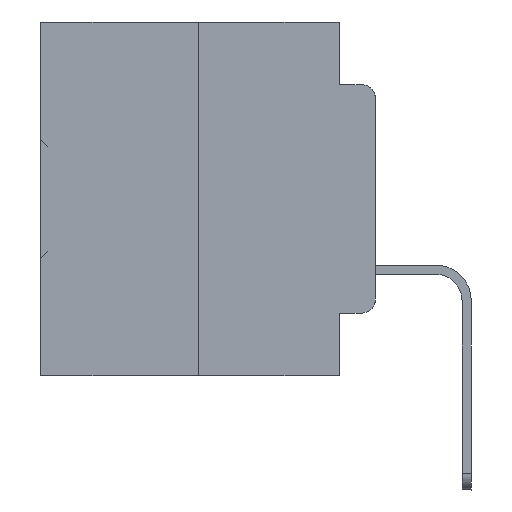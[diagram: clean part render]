
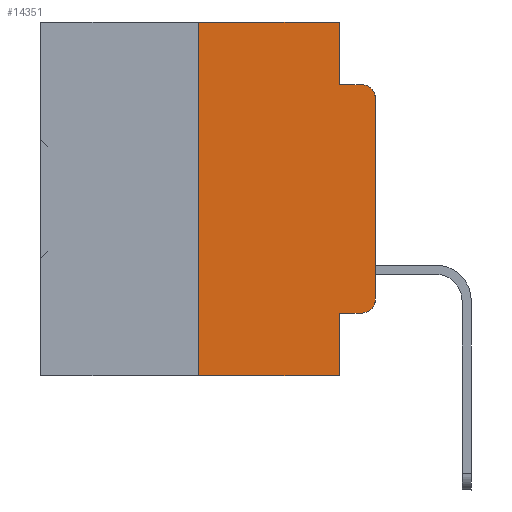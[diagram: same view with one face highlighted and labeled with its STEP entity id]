
A CAD part, left-side view. The second image highlights one B-rep face of the part: STEP entity #14351.
In plain terms, the highlighted planar face has unit normal (-1, 0, 0).
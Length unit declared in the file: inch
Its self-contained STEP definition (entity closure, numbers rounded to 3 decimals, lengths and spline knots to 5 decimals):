
#464 = ORIENTED_EDGE ( 'NONE', *, *, #23329, .T. ) ;
#886 = ORIENTED_EDGE ( 'NONE', *, *, #34393, .F. ) ;
#1000 = VECTOR ( 'NONE', #26115, 39.37008 ) ;
#1060 = DIRECTION ( 'NONE',  ( 1., 0., 0. ) ) ;
#1064 = EDGE_CURVE ( 'NONE', #6310, #15468, #34824, .T. ) ;
#1260 = CARTESIAN_POINT ( 'NONE',  ( 0., 0., -0.3915 ) ) ;
#1448 = EDGE_CURVE ( 'NONE', #9659, #15468, #21006, .T. ) ;
#2629 = CARTESIAN_POINT ( 'NONE',  ( 0., 0., 0. ) ) ;
#3159 = CARTESIAN_POINT ( 'NONE',  ( 0., 0.051, -0.4115 ) ) ;
#3976 = DIRECTION ( 'NONE',  ( 0., 0., -1. ) ) ;
#4759 = VECTOR ( 'NONE', #23052, 39.37008 ) ;
#5926 = LINE ( 'NONE', #27446, #6822 ) ;
#6259 = CARTESIAN_POINT ( 'NONE',  ( 0., 0.25, 0. ) ) ;
#6310 = VERTEX_POINT ( 'NONE', #32224 ) ;
#6533 = VERTEX_POINT ( 'NONE', #1260 ) ;
#6822 = VECTOR ( 'NONE', #21962, 39.37008 ) ;
#7250 = VECTOR ( 'NONE', #16641, 39.37008 ) ;
#7340 = AXIS2_PLACEMENT_3D ( 'NONE', #12041, #34841, #23015 ) ;
#7462 = CARTESIAN_POINT ( 'NONE',  ( 0., 0.051, -0.5 ) ) ;
#7631 = AXIS2_PLACEMENT_3D ( 'NONE', #33790, #19099, #10659 ) ;
#7667 = ORIENTED_EDGE ( 'NONE', *, *, #1448, .F. ) ;
#9610 = VERTEX_POINT ( 'NONE', #25015 ) ;
#9659 = VERTEX_POINT ( 'NONE', #11659 ) ;
#10255 = EDGE_CURVE ( 'NONE', #28352, #19261, #27536, .T. ) ;
#10659 = DIRECTION ( 'NONE',  ( 0., 0., -1. ) ) ;
#10896 = VECTOR ( 'NONE', #3976, 39.37008 ) ;
#10937 = ORIENTED_EDGE ( 'NONE', *, *, #1064, .T. ) ;
#10973 = EDGE_CURVE ( 'NONE', #26378, #19261, #30560, .T. ) ;
#11069 = EDGE_CURVE ( 'NONE', #28352, #28227, #15856, .T. ) ;
#11555 = CARTESIAN_POINT ( 'NONE',  ( 0., 0.051, -0.0885 ) ) ;
#11659 = CARTESIAN_POINT ( 'NONE',  ( 0., 0.051, -0.0885 ) ) ;
#12041 = CARTESIAN_POINT ( 'NONE',  ( 0., 0.02, -0.3915 ) ) ;
#12244 = ORIENTED_EDGE ( 'NONE', *, *, #10973, .F. ) ;
#12335 = DIRECTION ( 'NONE',  ( 0., 0., -1. ) ) ;
#12779 = EDGE_CURVE ( 'NONE', #26378, #9610, #28202, .T. ) ;
#14351 = ADVANCED_FACE ( 'NONE', ( #19048 ), #32396, .F. ) ;
#14421 = CARTESIAN_POINT ( 'NONE',  ( 0., 0.051, 0. ) ) ;
#14818 = ORIENTED_EDGE ( 'NONE', *, *, #11069, .F. ) ;
#14938 = CARTESIAN_POINT ( 'NONE',  ( 0., 0.25, 0. ) ) ;
#15468 = VERTEX_POINT ( 'NONE', #23496 ) ;
#15586 = CIRCLE ( 'NONE', #7340, 0.02 ) ;
#15856 = LINE ( 'NONE', #6259, #16288 ) ;
#16288 = VECTOR ( 'NONE', #26157, 39.37008 ) ;
#16641 = DIRECTION ( 'NONE',  ( 0., 0., 1. ) ) ;
#17046 = DIRECTION ( 'NONE',  ( 0., -1., 0. ) ) ;
#18567 = VECTOR ( 'NONE', #36543, 39.37008 ) ;
#18695 = VERTEX_POINT ( 'NONE', #30697 ) ;
#19048 = FACE_OUTER_BOUND ( 'NONE', #27106, .T. ) ;
#19099 = DIRECTION ( 'NONE',  ( -1., 0., 0. ) ) ;
#19261 = VERTEX_POINT ( 'NONE', #7462 ) ;
#20248 = LINE ( 'NONE', #23746, #10896 ) ;
#20640 = VECTOR ( 'NONE', #17046, 39.37008 ) ;
#21006 = LINE ( 'NONE', #11555, #1000 ) ;
#21076 = AXIS2_PLACEMENT_3D ( 'NONE', #29399, #1060, #12335 ) ;
#21637 = ORIENTED_EDGE ( 'NONE', *, *, #12779, .T. ) ;
#21962 = DIRECTION ( 'NONE',  ( 0., -1., 0. ) ) ;
#23015 = DIRECTION ( 'NONE',  ( 0., 0., -1. ) ) ;
#23052 = DIRECTION ( 'NONE',  ( 0., 0., -1. ) ) ;
#23097 = ORIENTED_EDGE ( 'NONE', *, *, #35213, .F. ) ;
#23329 = EDGE_CURVE ( 'NONE', #6533, #6310, #36212, .T. ) ;
#23496 = CARTESIAN_POINT ( 'NONE',  ( 0., 0.02, -0.0885 ) ) ;
#23746 = CARTESIAN_POINT ( 'NONE',  ( 0., 0.051, 0. ) ) ;
#24341 = ORIENTED_EDGE ( 'NONE', *, *, #28715, .T. ) ;
#25015 = CARTESIAN_POINT ( 'NONE',  ( 0., 0.02, -0.4115 ) ) ;
#26115 = DIRECTION ( 'NONE',  ( 0., -1., 0. ) ) ;
#26157 = DIRECTION ( 'NONE',  ( 0., 0., 1. ) ) ;
#26378 = VERTEX_POINT ( 'NONE', #27313 ) ;
#27106 = EDGE_LOOP ( 'NONE', ( #464, #10937, #7667, #886, #23097, #14818, #30843, #12244, #21637, #24341 ) ) ;
#27313 = CARTESIAN_POINT ( 'NONE',  ( 0., 0.051, -0.4115 ) ) ;
#27406 = CARTESIAN_POINT ( 'NONE',  ( 0., 0.25, -0.5 ) ) ;
#27446 = CARTESIAN_POINT ( 'NONE',  ( 0., 0.473, 0. ) ) ;
#27536 = LINE ( 'NONE', #36776, #18567 ) ;
#28202 = LINE ( 'NONE', #3159, #20640 ) ;
#28227 = VERTEX_POINT ( 'NONE', #14938 ) ;
#28352 = VERTEX_POINT ( 'NONE', #27406 ) ;
#28715 = EDGE_CURVE ( 'NONE', #9610, #6533, #15586, .T. ) ;
#29399 = CARTESIAN_POINT ( 'NONE',  ( 0., 0.473, 0. ) ) ;
#30560 = LINE ( 'NONE', #14421, #4759 ) ;
#30697 = CARTESIAN_POINT ( 'NONE',  ( 0., 0.051, 0. ) ) ;
#30843 = ORIENTED_EDGE ( 'NONE', *, *, #10255, .T. ) ;
#32224 = CARTESIAN_POINT ( 'NONE',  ( 0., 0., -0.1085 ) ) ;
#32396 = PLANE ( 'NONE',  #21076 ) ;
#33790 = CARTESIAN_POINT ( 'NONE',  ( 0., 0.02, -0.1085 ) ) ;
#34393 = EDGE_CURVE ( 'NONE', #18695, #9659, #20248, .T. ) ;
#34824 = CIRCLE ( 'NONE', #7631, 0.02 ) ;
#34841 = DIRECTION ( 'NONE',  ( -1., 0., 0. ) ) ;
#35213 = EDGE_CURVE ( 'NONE', #28227, #18695, #5926, .T. ) ;
#36212 = LINE ( 'NONE', #2629, #7250 ) ;
#36543 = DIRECTION ( 'NONE',  ( 0., -1., 0. ) ) ;
#36776 = CARTESIAN_POINT ( 'NONE',  ( 0., 0.473, -0.5 ) ) ;
